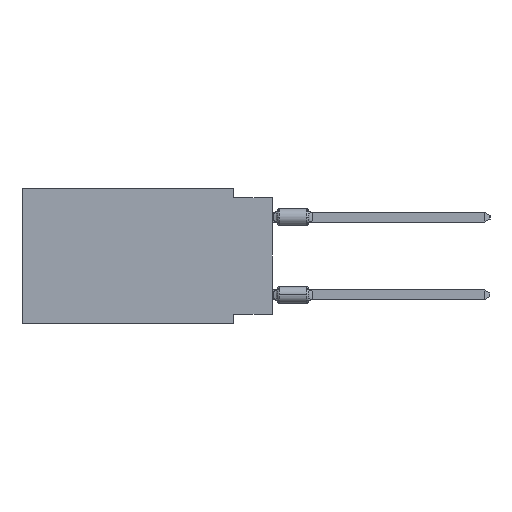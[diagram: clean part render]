
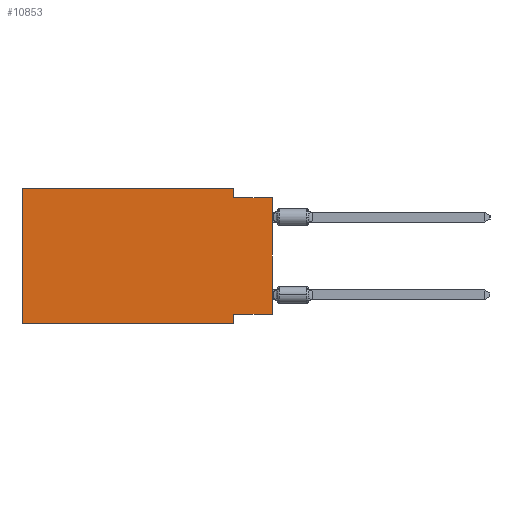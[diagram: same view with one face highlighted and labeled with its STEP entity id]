
A CAD part, left-side view. The second image highlights one B-rep face of the part: STEP entity #10853.
In plain terms, the highlighted planar face has unit normal (-1, 0, 0).
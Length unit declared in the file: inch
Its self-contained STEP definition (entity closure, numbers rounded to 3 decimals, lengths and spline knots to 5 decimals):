
#508 = CARTESIAN_POINT ( 'NONE',  ( 0., 0., 0. ) ) ;
#1969 = CARTESIAN_POINT ( 'NONE',  ( 0., 0.645, -0.35 ) ) ;
#3135 = VERTEX_POINT ( 'NONE', #42182 ) ;
#3283 = CARTESIAN_POINT ( 'NONE',  ( 0., 0.645, 0. ) ) ;
#3316 = CARTESIAN_POINT ( 'NONE',  ( 0., 0., -0.325 ) ) ;
#4032 = CARTESIAN_POINT ( 'NONE',  ( 0., 0., -0.025 ) ) ;
#4571 = VECTOR ( 'NONE', #56114, 39.37008 ) ;
#5375 = LINE ( 'NONE', #9459, #12543 ) ;
#5660 = DIRECTION ( 'NONE',  ( 1., 0., 0. ) ) ;
#6626 = LINE ( 'NONE', #508, #46570 ) ;
#7548 = CARTESIAN_POINT ( 'NONE',  ( 0., 0.1, -0.325 ) ) ;
#9459 = CARTESIAN_POINT ( 'NONE',  ( 0., 0.1, 0. ) ) ;
#10853 = ADVANCED_FACE ( 'NONE', ( #52293 ), #52624, .F. ) ;
#11825 = EDGE_CURVE ( 'NONE', #62293, #3135, #44501, .T. ) ;
#12164 = EDGE_CURVE ( 'NONE', #27851, #3135, #43070, .T. ) ;
#12543 = VECTOR ( 'NONE', #51331, 39.37008 ) ;
#16250 = VECTOR ( 'NONE', #44311, 39.37008 ) ;
#17176 = CARTESIAN_POINT ( 'NONE',  ( 0., 0.1, -0.025 ) ) ;
#17227 = DIRECTION ( 'NONE',  ( 0., 0., -1. ) ) ;
#18524 = DIRECTION ( 'NONE',  ( 0., -1., 0. ) ) ;
#18585 = VERTEX_POINT ( 'NONE', #24838 ) ;
#18858 = LINE ( 'NONE', #45374, #47456 ) ;
#20043 = LINE ( 'NONE', #4032, #35027 ) ;
#24838 = CARTESIAN_POINT ( 'NONE',  ( 0., 0.1, 0. ) ) ;
#25104 = VECTOR ( 'NONE', #17227, 39.37008 ) ;
#27081 = CARTESIAN_POINT ( 'NONE',  ( 0., 0.645, 0. ) ) ;
#27851 = VERTEX_POINT ( 'NONE', #7548 ) ;
#28176 = DIRECTION ( 'NONE',  ( 0., -1., 0. ) ) ;
#30031 = ORIENTED_EDGE ( 'NONE', *, *, #11825, .T. ) ;
#30344 = LINE ( 'NONE', #51114, #16250 ) ;
#31150 = DIRECTION ( 'NONE',  ( 0., 0., 1. ) ) ;
#31244 = ORIENTED_EDGE ( 'NONE', *, *, #52246, .F. ) ;
#32863 = ORIENTED_EDGE ( 'NONE', *, *, #67253, .T. ) ;
#33546 = EDGE_CURVE ( 'NONE', #44897, #27851, #30344, .T. ) ;
#33702 = AXIS2_PLACEMENT_3D ( 'NONE', #27081, #5660, #57742 ) ;
#34472 = CARTESIAN_POINT ( 'NONE',  ( 0., 0., -0.025 ) ) ;
#35027 = VECTOR ( 'NONE', #40785, 39.37008 ) ;
#37105 = EDGE_CURVE ( 'NONE', #62293, #38664, #60570, .T. ) ;
#37133 = EDGE_CURVE ( 'NONE', #40536, #50340, #20043, .T. ) ;
#38664 = VERTEX_POINT ( 'NONE', #3283 ) ;
#39370 = ORIENTED_EDGE ( 'NONE', *, *, #12164, .F. ) ;
#39395 = CARTESIAN_POINT ( 'NONE',  ( 0., 0.645, -0.35 ) ) ;
#39881 = ORIENTED_EDGE ( 'NONE', *, *, #33546, .F. ) ;
#40536 = VERTEX_POINT ( 'NONE', #17176 ) ;
#40785 = DIRECTION ( 'NONE',  ( 0., -1., 0. ) ) ;
#41635 = EDGE_LOOP ( 'NONE', ( #32863, #52261, #42452, #31244, #54295, #30031, #39370, #39881 ) ) ;
#41674 = EDGE_CURVE ( 'NONE', #18585, #40536, #5375, .T. ) ;
#42182 = CARTESIAN_POINT ( 'NONE',  ( 0., 0.1, -0.35 ) ) ;
#42452 = ORIENTED_EDGE ( 'NONE', *, *, #41674, .F. ) ;
#43070 = LINE ( 'NONE', #63870, #25104 ) ;
#44311 = DIRECTION ( 'NONE',  ( 0., 1., 0. ) ) ;
#44501 = LINE ( 'NONE', #39395, #62124 ) ;
#44897 = VERTEX_POINT ( 'NONE', #3316 ) ;
#45374 = CARTESIAN_POINT ( 'NONE',  ( 0., 0.645, 0. ) ) ;
#46570 = VECTOR ( 'NONE', #31150, 39.37008 ) ;
#47456 = VECTOR ( 'NONE', #18524, 39.37008 ) ;
#50340 = VERTEX_POINT ( 'NONE', #34472 ) ;
#51114 = CARTESIAN_POINT ( 'NONE',  ( 0., 0., -0.325 ) ) ;
#51331 = DIRECTION ( 'NONE',  ( 0., 0., -1. ) ) ;
#52246 = EDGE_CURVE ( 'NONE', #38664, #18585, #18858, .T. ) ;
#52261 = ORIENTED_EDGE ( 'NONE', *, *, #37133, .F. ) ;
#52293 = FACE_OUTER_BOUND ( 'NONE', #41635, .T. ) ;
#52624 = PLANE ( 'NONE',  #33702 ) ;
#54295 = ORIENTED_EDGE ( 'NONE', *, *, #37105, .F. ) ;
#55448 = CARTESIAN_POINT ( 'NONE',  ( 0., 0.645, 0. ) ) ;
#56114 = DIRECTION ( 'NONE',  ( 0., 0., 1. ) ) ;
#57742 = DIRECTION ( 'NONE',  ( 0., 0., -1. ) ) ;
#60570 = LINE ( 'NONE', #55448, #4571 ) ;
#62124 = VECTOR ( 'NONE', #28176, 39.37008 ) ;
#62293 = VERTEX_POINT ( 'NONE', #1969 ) ;
#63870 = CARTESIAN_POINT ( 'NONE',  ( 0., 0.1, -0.35 ) ) ;
#67253 = EDGE_CURVE ( 'NONE', #44897, #50340, #6626, .T. ) ;
